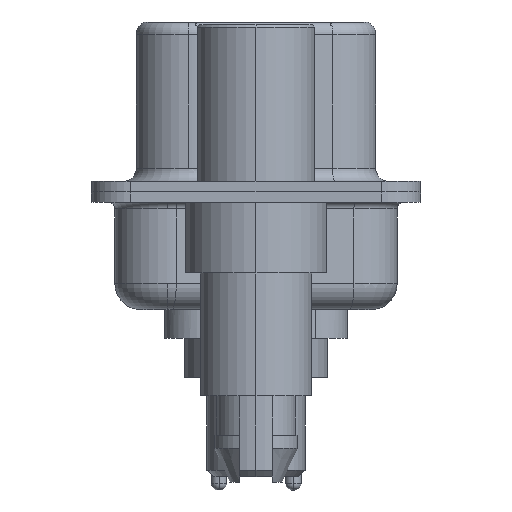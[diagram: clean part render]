
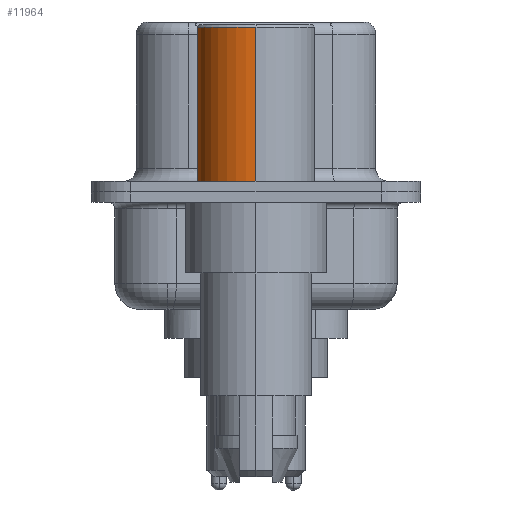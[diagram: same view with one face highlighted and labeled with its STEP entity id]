
A CAD part, left-side view. The second image highlights one B-rep face of the part: STEP entity #11964.
In plain terms, the highlighted cylindrical face has radius 2.25 mm (diameter 4.5 mm), a partial arc.
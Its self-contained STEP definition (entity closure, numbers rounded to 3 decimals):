
#509 = DIRECTION ( 'NONE',  ( 0., 0., 1. ) ) ;
#1174 = CYLINDRICAL_SURFACE ( 'NONE', #16746, 2.25 ) ;
#1200 = ORIENTED_EDGE ( 'NONE', *, *, #3044, .T. ) ;
#1286 = CIRCLE ( 'NONE', #2677, 2.25 ) ;
#1405 = CIRCLE ( 'NONE', #5496, 2.25 ) ;
#2677 = AXIS2_PLACEMENT_3D ( 'NONE', #7215, #5377, #5149 ) ;
#2865 = ORIENTED_EDGE ( 'NONE', *, *, #10130, .T. ) ;
#3014 = CARTESIAN_POINT ( 'NONE',  ( -2.25, 0., 0.4 ) ) ;
#3044 = EDGE_CURVE ( 'NONE', #17619, #23018, #1286, .T. ) ;
#3463 = ORIENTED_EDGE ( 'NONE', *, *, #22264, .F. ) ;
#4063 = CARTESIAN_POINT ( 'NONE',  ( -2.25, 0., 0.581 ) ) ;
#5149 = DIRECTION ( 'NONE',  ( 1., 0., 0. ) ) ;
#5377 = DIRECTION ( 'NONE',  ( 0., 0., 1. ) ) ;
#5496 = AXIS2_PLACEMENT_3D ( 'NONE', #6090, #18628, #7894 ) ;
#5816 = VECTOR ( 'NONE', #22812, 1000. ) ;
#5908 = EDGE_CURVE ( 'NONE', #17619, #16158, #11177, .T. ) ;
#6090 = CARTESIAN_POINT ( 'NONE',  ( 0., 0., 6.3 ) ) ;
#6437 = CARTESIAN_POINT ( 'NONE',  ( 2.25, 0., 0.4 ) ) ;
#7215 = CARTESIAN_POINT ( 'NONE',  ( 0., 0., 0.4 ) ) ;
#7458 = DIRECTION ( 'NONE',  ( 0., 0., 1. ) ) ;
#7661 = CARTESIAN_POINT ( 'NONE',  ( 2.25, 0., 6.3 ) ) ;
#7894 = DIRECTION ( 'NONE',  ( 1., 0., 0. ) ) ;
#9251 = DIRECTION ( 'NONE',  ( 1., 0., 0. ) ) ;
#10130 = EDGE_CURVE ( 'NONE', #23018, #17844, #12450, .T. ) ;
#10553 = EDGE_LOOP ( 'NONE', ( #1200, #2865, #3463, #16921 ) ) ;
#11177 = LINE ( 'NONE', #15800, #5816 ) ;
#11964 = ADVANCED_FACE ( 'NONE', ( #20158 ), #1174, .T. ) ;
#12450 = LINE ( 'NONE', #4063, #21319 ) ;
#15800 = CARTESIAN_POINT ( 'NONE',  ( 2.25, 0., 0.581 ) ) ;
#15952 = CARTESIAN_POINT ( 'NONE',  ( -2.25, 0., 6.3 ) ) ;
#16158 = VERTEX_POINT ( 'NONE', #7661 ) ;
#16746 = AXIS2_PLACEMENT_3D ( 'NONE', #21684, #7458, #9251 ) ;
#16921 = ORIENTED_EDGE ( 'NONE', *, *, #5908, .F. ) ;
#17619 = VERTEX_POINT ( 'NONE', #6437 ) ;
#17844 = VERTEX_POINT ( 'NONE', #15952 ) ;
#18628 = DIRECTION ( 'NONE',  ( 0., 0., 1. ) ) ;
#20158 = FACE_OUTER_BOUND ( 'NONE', #10553, .T. ) ;
#21319 = VECTOR ( 'NONE', #509, 1000. ) ;
#21684 = CARTESIAN_POINT ( 'NONE',  ( 0., 0., 0.581 ) ) ;
#22264 = EDGE_CURVE ( 'NONE', #16158, #17844, #1405, .T. ) ;
#22812 = DIRECTION ( 'NONE',  ( 0., 0., 1. ) ) ;
#23018 = VERTEX_POINT ( 'NONE', #3014 ) ;
